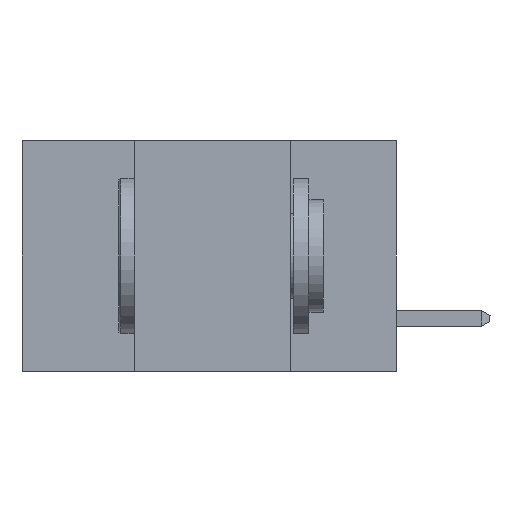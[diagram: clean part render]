
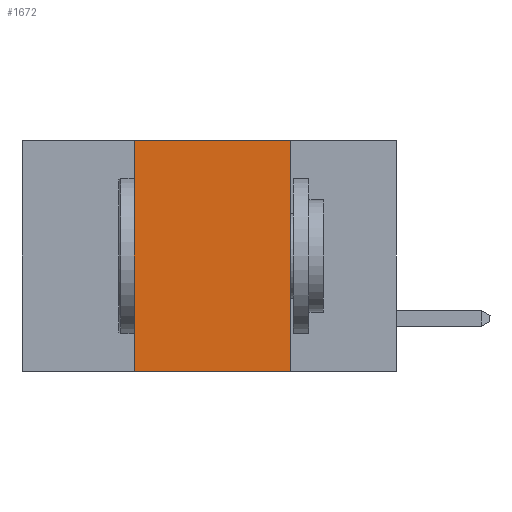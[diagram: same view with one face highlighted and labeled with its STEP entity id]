
A CAD part, left-side view. The second image highlights one B-rep face of the part: STEP entity #1672.
In plain terms, the highlighted planar face has unit normal (-1, 0, 0).
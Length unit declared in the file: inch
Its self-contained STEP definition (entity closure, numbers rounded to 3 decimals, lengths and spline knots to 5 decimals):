
#86 = DIRECTION ( 'NONE',  ( 0., 0., -1. ) ) ;
#578 = EDGE_LOOP ( 'NONE', ( #4744, #889, #695, #5086 ) ) ;
#695 = ORIENTED_EDGE ( 'NONE', *, *, #1853, .F. ) ;
#726 = PLANE ( 'NONE',  #4739 ) ;
#745 = EDGE_CURVE ( 'NONE', #2793, #10445, #867, .T. ) ;
#867 = LINE ( 'NONE', #6366, #2758 ) ;
#889 = ORIENTED_EDGE ( 'NONE', *, *, #3658, .F. ) ;
#1184 = CARTESIAN_POINT ( 'NONE',  ( 0., 0.17, -0.37 ) ) ;
#1334 = CARTESIAN_POINT ( 'NONE',  ( 0., 0.42, 0. ) ) ;
#1672 = ADVANCED_FACE ( 'NONE', ( #8405 ), #726, .F. ) ;
#1796 = VERTEX_POINT ( 'NONE', #1334 ) ;
#1853 = EDGE_CURVE ( 'NONE', #2793, #1796, #9909, .T. ) ;
#2551 = CARTESIAN_POINT ( 'NONE',  ( 0., 0.17, -0.37 ) ) ;
#2758 = VECTOR ( 'NONE', #2876, 39.37008 ) ;
#2793 = VERTEX_POINT ( 'NONE', #6908 ) ;
#2876 = DIRECTION ( 'NONE',  ( 0., -1., 0. ) ) ;
#3125 = DIRECTION ( 'NONE',  ( 0., 0., 1. ) ) ;
#3634 = LINE ( 'NONE', #2551, #9269 ) ;
#3658 = EDGE_CURVE ( 'NONE', #1796, #8826, #3842, .T. ) ;
#3842 = LINE ( 'NONE', #4575, #8351 ) ;
#3866 = CARTESIAN_POINT ( 'NONE',  ( 0., 0.42, -0.37 ) ) ;
#4151 = CARTESIAN_POINT ( 'NONE',  ( 0., 0.6, 0. ) ) ;
#4575 = CARTESIAN_POINT ( 'NONE',  ( 0., 0.6, 0. ) ) ;
#4739 = AXIS2_PLACEMENT_3D ( 'NONE', #4151, #9536, #8001 ) ;
#4744 = ORIENTED_EDGE ( 'NONE', *, *, #4876, .F. ) ;
#4876 = EDGE_CURVE ( 'NONE', #8826, #10445, #3634, .T. ) ;
#5086 = ORIENTED_EDGE ( 'NONE', *, *, #745, .T. ) ;
#5425 = DIRECTION ( 'NONE',  ( 0., -1., 0. ) ) ;
#6309 = CARTESIAN_POINT ( 'NONE',  ( 0., 0.17, 0. ) ) ;
#6366 = CARTESIAN_POINT ( 'NONE',  ( 0., 0.6, -0.37 ) ) ;
#6908 = CARTESIAN_POINT ( 'NONE',  ( 0., 0.42, -0.37 ) ) ;
#8001 = DIRECTION ( 'NONE',  ( 0., 0., -1. ) ) ;
#8351 = VECTOR ( 'NONE', #5425, 39.37008 ) ;
#8405 = FACE_OUTER_BOUND ( 'NONE', #578, .T. ) ;
#8826 = VERTEX_POINT ( 'NONE', #6309 ) ;
#9269 = VECTOR ( 'NONE', #86, 39.37008 ) ;
#9536 = DIRECTION ( 'NONE',  ( 1., 0., 0. ) ) ;
#9909 = LINE ( 'NONE', #3866, #10296 ) ;
#10296 = VECTOR ( 'NONE', #3125, 39.37008 ) ;
#10445 = VERTEX_POINT ( 'NONE', #1184 ) ;
